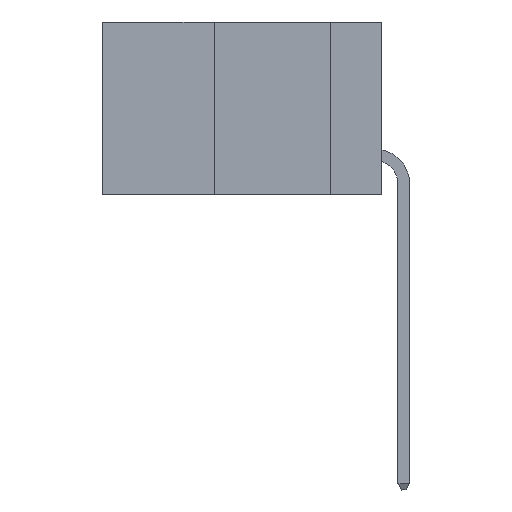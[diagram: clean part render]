
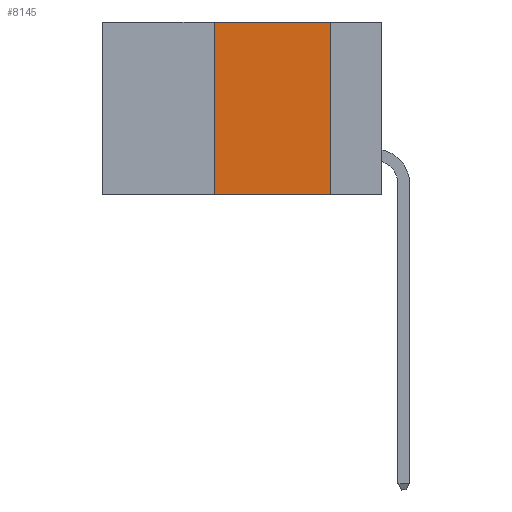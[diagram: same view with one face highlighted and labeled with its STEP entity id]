
A CAD part, left-side view. The second image highlights one B-rep face of the part: STEP entity #8145.
In plain terms, the highlighted planar face has unit normal (-1, 0, 0).
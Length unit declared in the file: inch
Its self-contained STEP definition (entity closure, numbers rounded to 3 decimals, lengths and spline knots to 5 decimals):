
#661 = CARTESIAN_POINT ( 'NONE',  ( 0., 0.11, -0.37 ) ) ;
#2768 = DIRECTION ( 'NONE',  ( 0., 0., -1. ) ) ;
#2933 = DIRECTION ( 'NONE',  ( 0., 0., 1. ) ) ;
#4881 = VECTOR ( 'NONE', #2933, 39.37008 ) ;
#7267 = CARTESIAN_POINT ( 'NONE',  ( 0., 0.6, 0. ) ) ;
#7774 = VECTOR ( 'NONE', #48719, 39.37008 ) ;
#8145 = ADVANCED_FACE ( 'NONE', ( #37114 ), #15298, .F. ) ;
#8202 = ORIENTED_EDGE ( 'NONE', *, *, #39804, .F. ) ;
#8932 = VECTOR ( 'NONE', #41158, 39.37008 ) ;
#12888 = VERTEX_POINT ( 'NONE', #661 ) ;
#13848 = VERTEX_POINT ( 'NONE', #26144 ) ;
#13961 = CARTESIAN_POINT ( 'NONE',  ( 0., 0.36, 0. ) ) ;
#14084 = CARTESIAN_POINT ( 'NONE',  ( 0., 0.6, -0.37 ) ) ;
#15298 = PLANE ( 'NONE',  #38194 ) ;
#17730 = LINE ( 'NONE', #13961, #4881 ) ;
#19797 = LINE ( 'NONE', #31315, #31832 ) ;
#25633 = LINE ( 'NONE', #14084, #8932 ) ;
#26144 = CARTESIAN_POINT ( 'NONE',  ( 0., 0.36, -0.37 ) ) ;
#28911 = VERTEX_POINT ( 'NONE', #34631 ) ;
#29092 = VERTEX_POINT ( 'NONE', #48598 ) ;
#31315 = CARTESIAN_POINT ( 'NONE',  ( 0., 0.6, 0. ) ) ;
#31802 = EDGE_CURVE ( 'NONE', #29092, #28911, #19797, .T. ) ;
#31832 = VECTOR ( 'NONE', #35081, 39.37008 ) ;
#33140 = ORIENTED_EDGE ( 'NONE', *, *, #38844, .T. ) ;
#34624 = LINE ( 'NONE', #40471, #7774 ) ;
#34631 = CARTESIAN_POINT ( 'NONE',  ( 0., 0.11, 0. ) ) ;
#35081 = DIRECTION ( 'NONE',  ( 0., -1., 0. ) ) ;
#37114 = FACE_OUTER_BOUND ( 'NONE', #39794, .T. ) ;
#38194 = AXIS2_PLACEMENT_3D ( 'NONE', #7267, #49388, #2768 ) ;
#38844 = EDGE_CURVE ( 'NONE', #13848, #12888, #25633, .T. ) ;
#39794 = EDGE_LOOP ( 'NONE', ( #44820, #49190, #8202, #33140 ) ) ;
#39804 = EDGE_CURVE ( 'NONE', #13848, #29092, #17730, .T. ) ;
#40471 = CARTESIAN_POINT ( 'NONE',  ( 0., 0.11, 0. ) ) ;
#41158 = DIRECTION ( 'NONE',  ( 0., -1., 0. ) ) ;
#44820 = ORIENTED_EDGE ( 'NONE', *, *, #45171, .F. ) ;
#45171 = EDGE_CURVE ( 'NONE', #28911, #12888, #34624, .T. ) ;
#48598 = CARTESIAN_POINT ( 'NONE',  ( 0., 0.36, 0. ) ) ;
#48719 = DIRECTION ( 'NONE',  ( 0., 0., -1. ) ) ;
#49190 = ORIENTED_EDGE ( 'NONE', *, *, #31802, .F. ) ;
#49388 = DIRECTION ( 'NONE',  ( 1., 0., 0. ) ) ;
